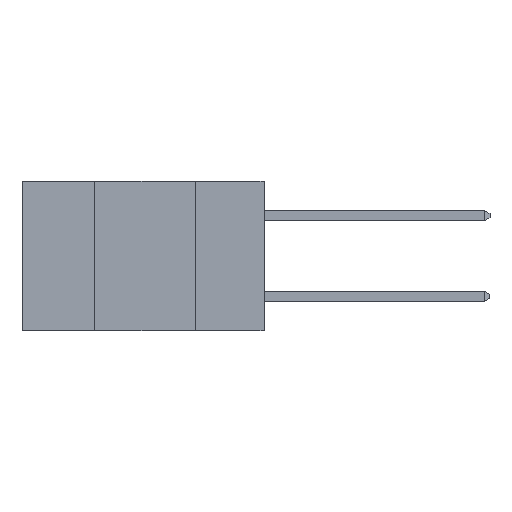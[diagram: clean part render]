
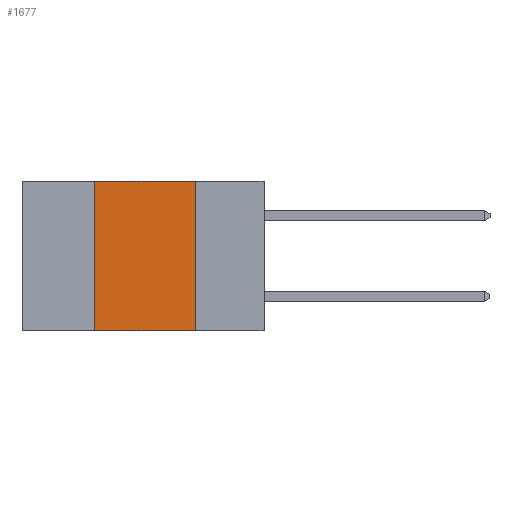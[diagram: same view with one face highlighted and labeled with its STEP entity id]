
A CAD part, left-side view. The second image highlights one B-rep face of the part: STEP entity #1677.
In plain terms, the highlighted planar face has unit normal (-1, 0, 0).
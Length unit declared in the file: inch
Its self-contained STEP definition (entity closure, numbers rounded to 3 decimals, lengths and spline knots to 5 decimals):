
#193 = VERTEX_POINT ( 'NONE', #8405 ) ;
#556 = VECTOR ( 'NONE', #11338, 39.37008 ) ;
#1285 = CARTESIAN_POINT ( 'NONE',  ( 0., 0.6, -0.37 ) ) ;
#1389 = VERTEX_POINT ( 'NONE', #3479 ) ;
#1677 = ADVANCED_FACE ( 'NONE', ( #6103 ), #5200, .F. ) ;
#1711 = LINE ( 'NONE', #2804, #6308 ) ;
#2707 = LINE ( 'NONE', #4811, #556 ) ;
#2804 = CARTESIAN_POINT ( 'NONE',  ( 0., 0.6, 0. ) ) ;
#3312 = DIRECTION ( 'NONE',  ( 0., 0., -1. ) ) ;
#3479 = CARTESIAN_POINT ( 'NONE',  ( 0., 0.42, 0. ) ) ;
#3731 = DIRECTION ( 'NONE',  ( 0., -1., 0. ) ) ;
#3996 = CARTESIAN_POINT ( 'NONE',  ( 0., 0.6, 0. ) ) ;
#4163 = CARTESIAN_POINT ( 'NONE',  ( 0., 0.17, 0. ) ) ;
#4266 = EDGE_CURVE ( 'NONE', #5123, #9575, #11120, .T. ) ;
#4468 = CARTESIAN_POINT ( 'NONE',  ( 0., 0.17, -0.37 ) ) ;
#4811 = CARTESIAN_POINT ( 'NONE',  ( 0., 0.42, 0. ) ) ;
#5115 = LINE ( 'NONE', #4163, #9833 ) ;
#5123 = VERTEX_POINT ( 'NONE', #11643 ) ;
#5200 = PLANE ( 'NONE',  #9363 ) ;
#5370 = EDGE_CURVE ( 'NONE', #1389, #193, #1711, .T. ) ;
#5495 = EDGE_CURVE ( 'NONE', #5123, #1389, #2707, .T. ) ;
#6068 = DIRECTION ( 'NONE',  ( 1., 0., 0. ) ) ;
#6103 = FACE_OUTER_BOUND ( 'NONE', #9453, .T. ) ;
#6308 = VECTOR ( 'NONE', #3731, 39.37008 ) ;
#6630 = ORIENTED_EDGE ( 'NONE', *, *, #8045, .F. ) ;
#6695 = ORIENTED_EDGE ( 'NONE', *, *, #5370, .F. ) ;
#6709 = ORIENTED_EDGE ( 'NONE', *, *, #5495, .F. ) ;
#6746 = ORIENTED_EDGE ( 'NONE', *, *, #4266, .T. ) ;
#8045 = EDGE_CURVE ( 'NONE', #193, #9575, #5115, .T. ) ;
#8405 = CARTESIAN_POINT ( 'NONE',  ( 0., 0.17, 0. ) ) ;
#8721 = VECTOR ( 'NONE', #9624, 39.37008 ) ;
#9363 = AXIS2_PLACEMENT_3D ( 'NONE', #3996, #6068, #3312 ) ;
#9453 = EDGE_LOOP ( 'NONE', ( #6630, #6695, #6709, #6746 ) ) ;
#9575 = VERTEX_POINT ( 'NONE', #4468 ) ;
#9624 = DIRECTION ( 'NONE',  ( 0., -1., 0. ) ) ;
#9833 = VECTOR ( 'NONE', #10674, 39.37008 ) ;
#10674 = DIRECTION ( 'NONE',  ( 0., 0., -1. ) ) ;
#11120 = LINE ( 'NONE', #1285, #8721 ) ;
#11338 = DIRECTION ( 'NONE',  ( 0., 0., 1. ) ) ;
#11643 = CARTESIAN_POINT ( 'NONE',  ( 0., 0.42, -0.37 ) ) ;
